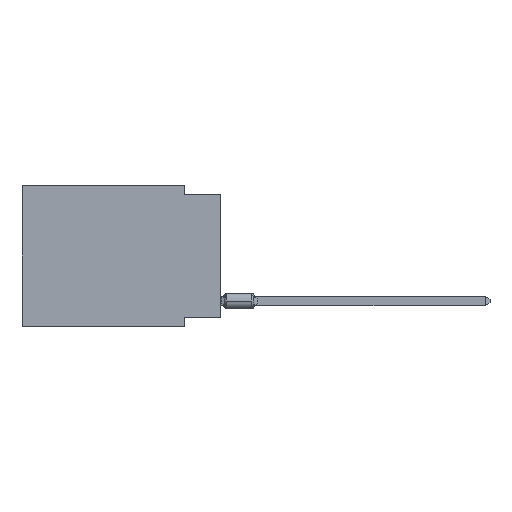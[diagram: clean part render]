
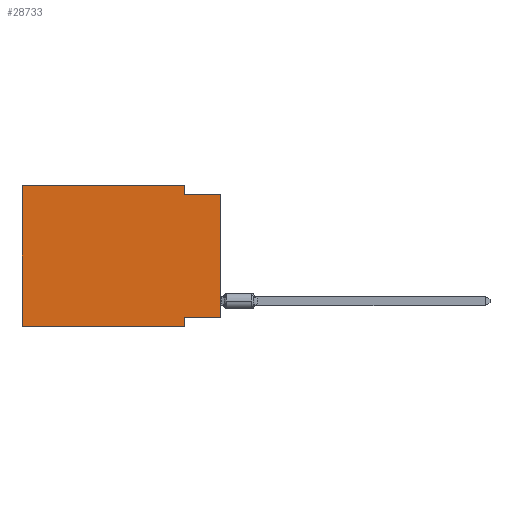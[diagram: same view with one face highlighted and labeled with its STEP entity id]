
A CAD part, left-side view. The second image highlights one B-rep face of the part: STEP entity #28733.
In plain terms, the highlighted planar face has unit normal (-1, 0, 0).
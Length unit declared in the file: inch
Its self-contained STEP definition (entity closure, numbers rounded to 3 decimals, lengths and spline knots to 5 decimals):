
#1229 = DIRECTION ( 'NONE',  ( 0., -1., 0. ) ) ;
#3538 = ORIENTED_EDGE ( 'NONE', *, *, #9385, .T. ) ;
#4000 = VECTOR ( 'NONE', #50521, 39.37008 ) ;
#4439 = LINE ( 'NONE', #9734, #49169 ) ;
#5656 = PLANE ( 'NONE',  #50631 ) ;
#6013 = CARTESIAN_POINT ( 'NONE',  ( 0., 0.1, 0. ) ) ;
#6023 = ORIENTED_EDGE ( 'NONE', *, *, #21432, .F. ) ;
#6593 = VECTOR ( 'NONE', #42159, 39.37008 ) ;
#9385 = EDGE_CURVE ( 'NONE', #37624, #22459, #22940, .T. ) ;
#9734 = CARTESIAN_POINT ( 'NONE',  ( 0., 0., 0. ) ) ;
#12696 = VERTEX_POINT ( 'NONE', #22423 ) ;
#13540 = CARTESIAN_POINT ( 'NONE',  ( 0., 0.55, 0. ) ) ;
#13673 = LINE ( 'NONE', #46525, #27016 ) ;
#14613 = FACE_OUTER_BOUND ( 'NONE', #38824, .T. ) ;
#15101 = DIRECTION ( 'NONE',  ( 0., -1., 0. ) ) ;
#15619 = ORIENTED_EDGE ( 'NONE', *, *, #35881, .F. ) ;
#16442 = CARTESIAN_POINT ( 'NONE',  ( 0., 0.1, -0.39 ) ) ;
#16996 = CARTESIAN_POINT ( 'NONE',  ( 0., 0.1, 0. ) ) ;
#19351 = CARTESIAN_POINT ( 'NONE',  ( 0., 0.55, 0. ) ) ;
#20828 = DIRECTION ( 'NONE',  ( 0., 0., 1. ) ) ;
#21432 = EDGE_CURVE ( 'NONE', #25502, #46413, #52793, .T. ) ;
#22423 = CARTESIAN_POINT ( 'NONE',  ( 0., 0.55, 0. ) ) ;
#22459 = VERTEX_POINT ( 'NONE', #34597 ) ;
#22686 = CARTESIAN_POINT ( 'NONE',  ( 0., 0.1, -0.025 ) ) ;
#22764 = EDGE_CURVE ( 'NONE', #26117, #22459, #54697, .T. ) ;
#22940 = LINE ( 'NONE', #53099, #29872 ) ;
#23467 = VERTEX_POINT ( 'NONE', #42239 ) ;
#23533 = CARTESIAN_POINT ( 'NONE',  ( 0., 0., -0.365 ) ) ;
#23575 = ORIENTED_EDGE ( 'NONE', *, *, #45524, .T. ) ;
#25502 = VERTEX_POINT ( 'NONE', #6013 ) ;
#26117 = VERTEX_POINT ( 'NONE', #39116 ) ;
#27016 = VECTOR ( 'NONE', #20828, 39.37008 ) ;
#28733 = ADVANCED_FACE ( 'NONE', ( #14613 ), #5656, .F. ) ;
#29872 = VECTOR ( 'NONE', #15101, 39.37008 ) ;
#30939 = LINE ( 'NONE', #42970, #51467 ) ;
#31124 = DIRECTION ( 'NONE',  ( 1., 0., 0. ) ) ;
#31488 = VECTOR ( 'NONE', #1229, 39.37008 ) ;
#31674 = DIRECTION ( 'NONE',  ( 0., 0., -1. ) ) ;
#32507 = VERTEX_POINT ( 'NONE', #52158 ) ;
#33841 = EDGE_CURVE ( 'NONE', #37624, #12696, #13673, .T. ) ;
#34032 = EDGE_CURVE ( 'NONE', #12696, #25502, #52378, .T. ) ;
#34597 = CARTESIAN_POINT ( 'NONE',  ( 0., 0.1, -0.39 ) ) ;
#35881 = EDGE_CURVE ( 'NONE', #23467, #26117, #36380, .T. ) ;
#36380 = LINE ( 'NONE', #23533, #40530 ) ;
#36777 = ORIENTED_EDGE ( 'NONE', *, *, #33841, .F. ) ;
#37207 = CARTESIAN_POINT ( 'NONE',  ( 0., 0.55, -0.39 ) ) ;
#37624 = VERTEX_POINT ( 'NONE', #37207 ) ;
#38824 = EDGE_LOOP ( 'NONE', ( #23575, #46450, #6023, #51888, #36777, #3538, #48799, #15619 ) ) ;
#39116 = CARTESIAN_POINT ( 'NONE',  ( 0., 0.1, -0.365 ) ) ;
#40530 = VECTOR ( 'NONE', #53686, 39.37008 ) ;
#42159 = DIRECTION ( 'NONE',  ( 0., 0., -1. ) ) ;
#42239 = CARTESIAN_POINT ( 'NONE',  ( 0., 0., -0.365 ) ) ;
#42758 = DIRECTION ( 'NONE',  ( 0., 0., 1. ) ) ;
#42970 = CARTESIAN_POINT ( 'NONE',  ( 0., 0., -0.025 ) ) ;
#45524 = EDGE_CURVE ( 'NONE', #23467, #32507, #4439, .T. ) ;
#46413 = VERTEX_POINT ( 'NONE', #22686 ) ;
#46450 = ORIENTED_EDGE ( 'NONE', *, *, #47150, .F. ) ;
#46525 = CARTESIAN_POINT ( 'NONE',  ( 0., 0.55, 0. ) ) ;
#47150 = EDGE_CURVE ( 'NONE', #46413, #32507, #30939, .T. ) ;
#47423 = DIRECTION ( 'NONE',  ( 0., -1., 0. ) ) ;
#48799 = ORIENTED_EDGE ( 'NONE', *, *, #22764, .F. ) ;
#49169 = VECTOR ( 'NONE', #42758, 39.37008 ) ;
#50521 = DIRECTION ( 'NONE',  ( 0., 0., -1. ) ) ;
#50631 = AXIS2_PLACEMENT_3D ( 'NONE', #19351, #31124, #31674 ) ;
#51467 = VECTOR ( 'NONE', #47423, 39.37008 ) ;
#51888 = ORIENTED_EDGE ( 'NONE', *, *, #34032, .F. ) ;
#52158 = CARTESIAN_POINT ( 'NONE',  ( 0., 0., -0.025 ) ) ;
#52378 = LINE ( 'NONE', #13540, #31488 ) ;
#52793 = LINE ( 'NONE', #16996, #6593 ) ;
#53099 = CARTESIAN_POINT ( 'NONE',  ( 0., 0.55, -0.39 ) ) ;
#53686 = DIRECTION ( 'NONE',  ( 0., 1., 0. ) ) ;
#54697 = LINE ( 'NONE', #16442, #4000 ) ;
